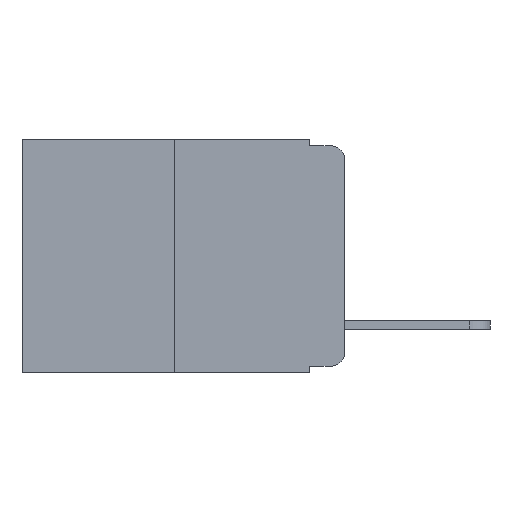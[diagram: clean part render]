
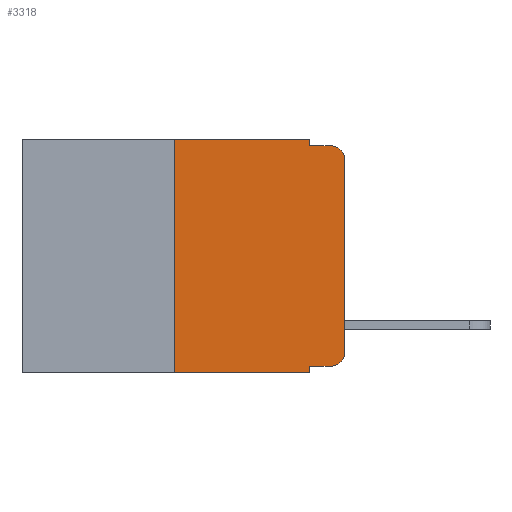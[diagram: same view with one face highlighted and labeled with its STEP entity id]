
A CAD part, left-side view. The second image highlights one B-rep face of the part: STEP entity #3318.
In plain terms, the highlighted planar face has unit normal (-1, 0, 0).
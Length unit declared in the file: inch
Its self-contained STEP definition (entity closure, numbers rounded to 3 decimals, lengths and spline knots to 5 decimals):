
#319 = FACE_OUTER_BOUND ( 'NONE', #2085, .T. ) ;
#456 = CARTESIAN_POINT ( 'NONE',  ( 0., 0.051, -0.343 ) ) ;
#507 = VECTOR ( 'NONE', #6675, 39.37008 ) ;
#879 = LINE ( 'NONE', #8761, #507 ) ;
#929 = DIRECTION ( 'NONE',  ( -1., 0., 0. ) ) ;
#1086 = VERTEX_POINT ( 'NONE', #456 ) ;
#1263 = VECTOR ( 'NONE', #9155, 39.37008 ) ;
#1282 = DIRECTION ( 'NONE',  ( 0., 0., 1. ) ) ;
#1326 = CARTESIAN_POINT ( 'NONE',  ( 0., 0.051, -0.01 ) ) ;
#1336 = LINE ( 'NONE', #11676, #1263 ) ;
#1490 = VERTEX_POINT ( 'NONE', #1919 ) ;
#1538 = DIRECTION ( 'NONE',  ( 0., -1., 0. ) ) ;
#1571 = CARTESIAN_POINT ( 'NONE',  ( 0., 0.25, 0. ) ) ;
#1919 = CARTESIAN_POINT ( 'NONE',  ( 0., 0., -0.313 ) ) ;
#2085 = EDGE_LOOP ( 'NONE', ( #8970, #9129, #9085, #9164, #4914, #3584, #9775, #9171, #9180, #9243 ) ) ;
#2443 = VERTEX_POINT ( 'NONE', #6590 ) ;
#2693 = CARTESIAN_POINT ( 'NONE',  ( 0., 0.473, 0. ) ) ;
#2925 = CARTESIAN_POINT ( 'NONE',  ( 0., 0.02, -0.313 ) ) ;
#2940 = CARTESIAN_POINT ( 'NONE',  ( 0., 0.051, -0.333 ) ) ;
#3318 = ADVANCED_FACE ( 'NONE', ( #319 ), #8945, .F. ) ;
#3320 = CARTESIAN_POINT ( 'NONE',  ( 0., 0.25, 0. ) ) ;
#3345 = CARTESIAN_POINT ( 'NONE',  ( 0., 0.02, -0.01 ) ) ;
#3584 = ORIENTED_EDGE ( 'NONE', *, *, #6761, .F. ) ;
#3621 = DIRECTION ( 'NONE',  ( -1., 0., 0. ) ) ;
#3799 = EDGE_CURVE ( 'NONE', #8641, #9701, #5853, .T. ) ;
#4643 = VERTEX_POINT ( 'NONE', #6696 ) ;
#4914 = ORIENTED_EDGE ( 'NONE', *, *, #3799, .F. ) ;
#5031 = VECTOR ( 'NONE', #12188, 39.37008 ) ;
#5090 = CIRCLE ( 'NONE', #10962, 0.02 ) ;
#5602 = EDGE_CURVE ( 'NONE', #2443, #1086, #1336, .T. ) ;
#5802 = VERTEX_POINT ( 'NONE', #3345 ) ;
#5853 = LINE ( 'NONE', #2693, #5031 ) ;
#6357 = CARTESIAN_POINT ( 'NONE',  ( 0., 0., -0.03 ) ) ;
#6590 = CARTESIAN_POINT ( 'NONE',  ( 0., 0.25, -0.343 ) ) ;
#6622 = EDGE_CURVE ( 'NONE', #1490, #8723, #9022, .T. ) ;
#6675 = DIRECTION ( 'NONE',  ( 0., 0., -1. ) ) ;
#6679 = EDGE_CURVE ( 'NONE', #8723, #5802, #8213, .T. ) ;
#6694 = EDGE_CURVE ( 'NONE', #9475, #5802, #7885, .T. ) ;
#6696 = CARTESIAN_POINT ( 'NONE',  ( 0., 0.02, -0.333 ) ) ;
#6709 = EDGE_CURVE ( 'NONE', #9701, #9475, #7876, .T. ) ;
#6761 = EDGE_CURVE ( 'NONE', #2443, #8641, #7034, .T. ) ;
#6872 = VECTOR ( 'NONE', #1282, 39.37008 ) ;
#7034 = LINE ( 'NONE', #1571, #6872 ) ;
#7133 = VERTEX_POINT ( 'NONE', #2940 ) ;
#7474 = CARTESIAN_POINT ( 'NONE',  ( 0., 0.473, 0. ) ) ;
#7637 = VECTOR ( 'NONE', #11675, 39.37008 ) ;
#7651 = DIRECTION ( 'NONE',  ( 0., 0., 1. ) ) ;
#7665 = CARTESIAN_POINT ( 'NONE',  ( 0., 0., 0. ) ) ;
#7873 = VECTOR ( 'NONE', #10206, 39.37008 ) ;
#7876 = LINE ( 'NONE', #8758, #7637 ) ;
#7885 = LINE ( 'NONE', #1326, #7873 ) ;
#8148 = AXIS2_PLACEMENT_3D ( 'NONE', #7474, #9736, #9733 ) ;
#8213 = CIRCLE ( 'NONE', #11317, 0.02 ) ;
#8641 = VERTEX_POINT ( 'NONE', #3320 ) ;
#8723 = VERTEX_POINT ( 'NONE', #6357 ) ;
#8758 = CARTESIAN_POINT ( 'NONE',  ( 0., 0.051, 0. ) ) ;
#8759 = VECTOR ( 'NONE', #7651, 39.37008 ) ;
#8761 = CARTESIAN_POINT ( 'NONE',  ( 0., 0.051, 0. ) ) ;
#8945 = PLANE ( 'NONE',  #8148 ) ;
#8970 = ORIENTED_EDGE ( 'NONE', *, *, #6622, .T. ) ;
#9022 = LINE ( 'NONE', #7665, #8759 ) ;
#9085 = ORIENTED_EDGE ( 'NONE', *, *, #6694, .F. ) ;
#9129 = ORIENTED_EDGE ( 'NONE', *, *, #6679, .T. ) ;
#9155 = DIRECTION ( 'NONE',  ( 0., -1., 0. ) ) ;
#9164 = ORIENTED_EDGE ( 'NONE', *, *, #6709, .F. ) ;
#9171 = ORIENTED_EDGE ( 'NONE', *, *, #10259, .F. ) ;
#9180 = ORIENTED_EDGE ( 'NONE', *, *, #10294, .T. ) ;
#9243 = ORIENTED_EDGE ( 'NONE', *, *, #10314, .T. ) ;
#9434 = CARTESIAN_POINT ( 'NONE',  ( 0., 0.051, -0.333 ) ) ;
#9475 = VERTEX_POINT ( 'NONE', #12147 ) ;
#9701 = VERTEX_POINT ( 'NONE', #10946 ) ;
#9733 = DIRECTION ( 'NONE',  ( 0., 0., -1. ) ) ;
#9736 = DIRECTION ( 'NONE',  ( 1., 0., 0. ) ) ;
#9775 = ORIENTED_EDGE ( 'NONE', *, *, #5602, .T. ) ;
#10117 = LINE ( 'NONE', #9434, #12072 ) ;
#10206 = DIRECTION ( 'NONE',  ( 0., -1., 0. ) ) ;
#10259 = EDGE_CURVE ( 'NONE', #7133, #1086, #879, .T. ) ;
#10294 = EDGE_CURVE ( 'NONE', #7133, #4643, #10117, .T. ) ;
#10314 = EDGE_CURVE ( 'NONE', #4643, #1490, #5090, .T. ) ;
#10456 = DIRECTION ( 'NONE',  ( 0., 0., -1. ) ) ;
#10946 = CARTESIAN_POINT ( 'NONE',  ( 0., 0.051, 0. ) ) ;
#10962 = AXIS2_PLACEMENT_3D ( 'NONE', #2925, #3621, #11442 ) ;
#11123 = CARTESIAN_POINT ( 'NONE',  ( 0., 0.02, -0.03 ) ) ;
#11317 = AXIS2_PLACEMENT_3D ( 'NONE', #11123, #929, #10456 ) ;
#11442 = DIRECTION ( 'NONE',  ( 0., 0., -1. ) ) ;
#11675 = DIRECTION ( 'NONE',  ( 0., 0., -1. ) ) ;
#11676 = CARTESIAN_POINT ( 'NONE',  ( 0., 0.473, -0.343 ) ) ;
#12072 = VECTOR ( 'NONE', #1538, 39.37008 ) ;
#12147 = CARTESIAN_POINT ( 'NONE',  ( 0., 0.051, -0.01 ) ) ;
#12188 = DIRECTION ( 'NONE',  ( 0., -1., 0. ) ) ;
